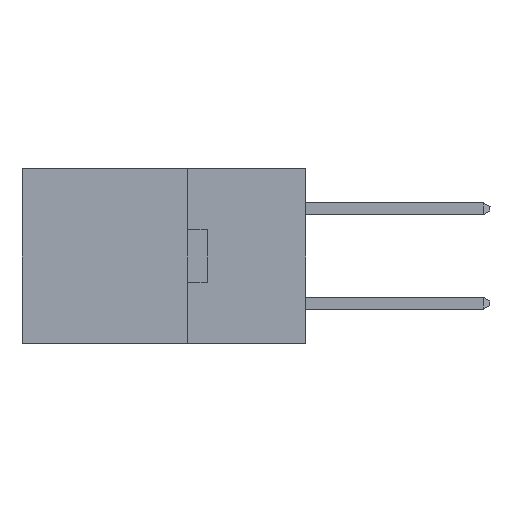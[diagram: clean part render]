
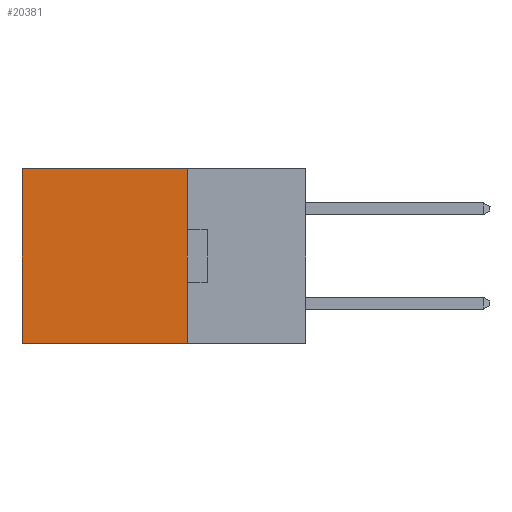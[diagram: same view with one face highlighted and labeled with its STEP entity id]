
A CAD part, left-side view. The second image highlights one B-rep face of the part: STEP entity #20381.
In plain terms, the highlighted planar face has unit normal (-1, 0, 0).
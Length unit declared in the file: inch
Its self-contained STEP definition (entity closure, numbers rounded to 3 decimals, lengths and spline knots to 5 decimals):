
#41 = DIRECTION ( 'NONE',  ( 0., 0., -1. ) ) ;
#51 = EDGE_LOOP ( 'NONE', ( #23928, #21282, #1191, #17458 ) ) ;
#812 = CARTESIAN_POINT ( 'NONE',  ( 0.2615, 0.6, -0.37 ) ) ;
#1191 = ORIENTED_EDGE ( 'NONE', *, *, #19320, .F. ) ;
#3685 = CARTESIAN_POINT ( 'NONE',  ( 0.2615, 0.25, -0.37 ) ) ;
#4479 = LINE ( 'NONE', #24239, #10363 ) ;
#4484 = VECTOR ( 'NONE', #7501, 39.37008 ) ;
#5583 = VECTOR ( 'NONE', #28073, 39.37008 ) ;
#5838 = LINE ( 'NONE', #812, #4484 ) ;
#5872 = DIRECTION ( 'NONE',  ( 0., 0., -1. ) ) ;
#6223 = CARTESIAN_POINT ( 'NONE',  ( 0.2615, 0.6, 0. ) ) ;
#7501 = DIRECTION ( 'NONE',  ( 0., 0., -1. ) ) ;
#7641 = VERTEX_POINT ( 'NONE', #23776 ) ;
#8739 = CARTESIAN_POINT ( 'NONE',  ( 0.2615, 0.25, 0. ) ) ;
#10363 = VECTOR ( 'NONE', #41, 39.37008 ) ;
#12986 = EDGE_CURVE ( 'NONE', #14053, #19852, #22747, .T. ) ;
#14053 = VERTEX_POINT ( 'NONE', #27173 ) ;
#16738 = PLANE ( 'NONE',  #24167 ) ;
#16969 = VECTOR ( 'NONE', #19664, 39.37008 ) ;
#17265 = LINE ( 'NONE', #23927, #5583 ) ;
#17458 = ORIENTED_EDGE ( 'NONE', *, *, #12986, .T. ) ;
#19033 = DIRECTION ( 'NONE',  ( 1., 0., 0. ) ) ;
#19320 = EDGE_CURVE ( 'NONE', #14053, #7641, #4479, .T. ) ;
#19664 = DIRECTION ( 'NONE',  ( 0., 1., 0. ) ) ;
#19852 = VERTEX_POINT ( 'NONE', #6223 ) ;
#19901 = EDGE_CURVE ( 'NONE', #7641, #22031, #17265, .T. ) ;
#20381 = ADVANCED_FACE ( 'NONE', ( #23098 ), #16738, .F. ) ;
#21282 = ORIENTED_EDGE ( 'NONE', *, *, #19901, .F. ) ;
#21477 = EDGE_CURVE ( 'NONE', #19852, #22031, #5838, .T. ) ;
#22031 = VERTEX_POINT ( 'NONE', #24481 ) ;
#22747 = LINE ( 'NONE', #8739, #16969 ) ;
#23098 = FACE_OUTER_BOUND ( 'NONE', #51, .T. ) ;
#23776 = CARTESIAN_POINT ( 'NONE',  ( 0.2615, 0.25, -0.37 ) ) ;
#23927 = CARTESIAN_POINT ( 'NONE',  ( 0.2615, 0.25, -0.37 ) ) ;
#23928 = ORIENTED_EDGE ( 'NONE', *, *, #21477, .T. ) ;
#24167 = AXIS2_PLACEMENT_3D ( 'NONE', #3685, #19033, #5872 ) ;
#24239 = CARTESIAN_POINT ( 'NONE',  ( 0.2615, 0.25, -0.37 ) ) ;
#24481 = CARTESIAN_POINT ( 'NONE',  ( 0.2615, 0.6, -0.37 ) ) ;
#27173 = CARTESIAN_POINT ( 'NONE',  ( 0.2615, 0.25, 0. ) ) ;
#28073 = DIRECTION ( 'NONE',  ( 0., 1., 0. ) ) ;
